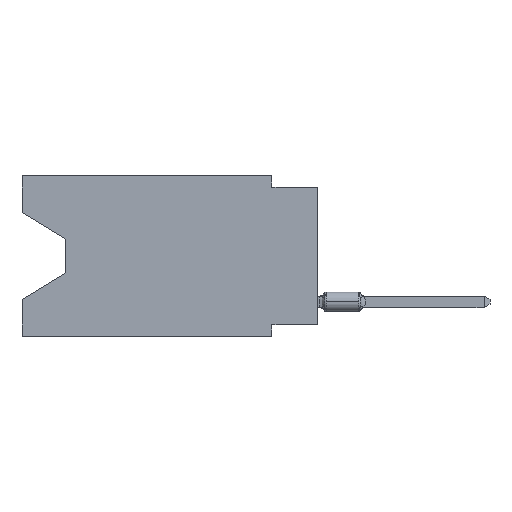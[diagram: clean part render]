
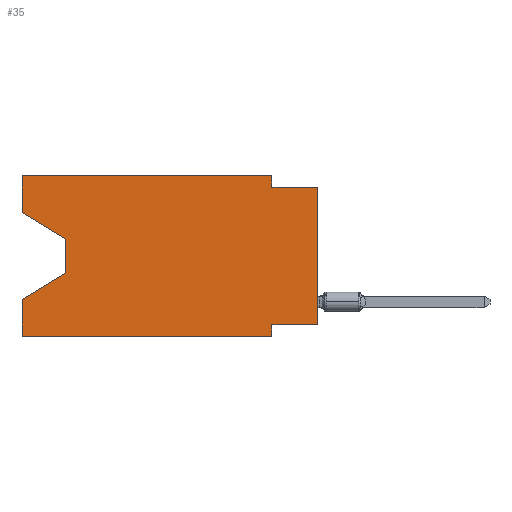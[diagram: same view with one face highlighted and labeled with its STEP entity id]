
A CAD part, left-side view. The second image highlights one B-rep face of the part: STEP entity #35.
In plain terms, the highlighted planar face has unit normal (-1, 0, 0).
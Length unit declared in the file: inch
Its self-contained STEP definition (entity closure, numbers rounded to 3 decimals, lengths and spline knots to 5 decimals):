
#35 = ADVANCED_FACE ( 'NONE', ( #199 ), #6060, .F. ) ;
#199 = FACE_OUTER_BOUND ( 'NONE', #285, .T. ) ;
#207 = VECTOR ( 'NONE', #5463, 39.37008 ) ;
#285 = EDGE_LOOP ( 'NONE', ( #1194, #2487, #8710, #9950, #14336, #1854, #3718, #14926, #2462, #6976, #872, #2185 ) ) ;
#323 = VECTOR ( 'NONE', #14289, 39.37008 ) ;
#442 = LINE ( 'NONE', #12983, #7200 ) ;
#547 = CARTESIAN_POINT ( 'NONE',  ( 0., 0.1, 0. ) ) ;
#564 = CARTESIAN_POINT ( 'NONE',  ( 0., 0.645, 0. ) ) ;
#569 = VERTEX_POINT ( 'NONE', #8991 ) ;
#685 = VECTOR ( 'NONE', #10960, 39.37008 ) ;
#872 = ORIENTED_EDGE ( 'NONE', *, *, #5659, .F. ) ;
#1194 = ORIENTED_EDGE ( 'NONE', *, *, #13750, .T. ) ;
#1289 = CARTESIAN_POINT ( 'NONE',  ( 0., 0., -0.325 ) ) ;
#1396 = LINE ( 'NONE', #14093, #13745 ) ;
#1601 = LINE ( 'NONE', #2672, #9532 ) ;
#1622 = DIRECTION ( 'NONE',  ( 0., 0., 1. ) ) ;
#1655 = DIRECTION ( 'NONE',  ( 0., 0., 1. ) ) ;
#1800 = VECTOR ( 'NONE', #10485, 39.37008 ) ;
#1826 = LINE ( 'NONE', #8537, #685 ) ;
#1854 = ORIENTED_EDGE ( 'NONE', *, *, #6015, .F. ) ;
#1916 = EDGE_CURVE ( 'NONE', #7897, #9151, #1601, .T. ) ;
#2185 = ORIENTED_EDGE ( 'NONE', *, *, #3210, .F. ) ;
#2310 = CARTESIAN_POINT ( 'NONE',  ( 0., 0.645, -0.35 ) ) ;
#2462 = ORIENTED_EDGE ( 'NONE', *, *, #7798, .F. ) ;
#2487 = ORIENTED_EDGE ( 'NONE', *, *, #11870, .T. ) ;
#2672 = CARTESIAN_POINT ( 'NONE',  ( 0., 0., -0.325 ) ) ;
#2851 = LINE ( 'NONE', #564, #5051 ) ;
#3210 = EDGE_CURVE ( 'NONE', #569, #8963, #8355, .T. ) ;
#3262 = DIRECTION ( 'NONE',  ( 0., -0.855, -0.519 ) ) ;
#3718 = ORIENTED_EDGE ( 'NONE', *, *, #1916, .F. ) ;
#3863 = DIRECTION ( 'NONE',  ( 1., 0., 0. ) ) ;
#3877 = CARTESIAN_POINT ( 'NONE',  ( 0., 0.1, -0.35 ) ) ;
#3897 = VERTEX_POINT ( 'NONE', #11573 ) ;
#4515 = EDGE_CURVE ( 'NONE', #5118, #12363, #7208, .T. ) ;
#5051 = VECTOR ( 'NONE', #1622, 39.37008 ) ;
#5079 = CARTESIAN_POINT ( 'NONE',  ( 0., 0.645, 0. ) ) ;
#5118 = VERTEX_POINT ( 'NONE', #2310 ) ;
#5463 = DIRECTION ( 'NONE',  ( 0., 0., -1. ) ) ;
#5659 = EDGE_CURVE ( 'NONE', #8963, #6902, #9208, .T. ) ;
#5695 = VERTEX_POINT ( 'NONE', #6234 ) ;
#6015 = EDGE_CURVE ( 'NONE', #9151, #12363, #12676, .T. ) ;
#6060 = PLANE ( 'NONE',  #7201 ) ;
#6234 = CARTESIAN_POINT ( 'NONE',  ( 0., 0.55, -0.212 ) ) ;
#6272 = VERTEX_POINT ( 'NONE', #9863 ) ;
#6749 = LINE ( 'NONE', #8810, #207 ) ;
#6893 = CARTESIAN_POINT ( 'NONE',  ( 0., 0.1, -0.35 ) ) ;
#6902 = VERTEX_POINT ( 'NONE', #547 ) ;
#6976 = ORIENTED_EDGE ( 'NONE', *, *, #12416, .F. ) ;
#7200 = VECTOR ( 'NONE', #1655, 39.37008 ) ;
#7201 = AXIS2_PLACEMENT_3D ( 'NONE', #5079, #3863, #14353 ) ;
#7208 = LINE ( 'NONE', #11852, #13923 ) ;
#7536 = EDGE_CURVE ( 'NONE', #5695, #6272, #1396, .T. ) ;
#7741 = VERTEX_POINT ( 'NONE', #12568 ) ;
#7798 = EDGE_CURVE ( 'NONE', #3897, #7741, #8850, .T. ) ;
#7897 = VERTEX_POINT ( 'NONE', #1289 ) ;
#8237 = CARTESIAN_POINT ( 'NONE',  ( 0., 0.1, -0.325 ) ) ;
#8319 = DIRECTION ( 'NONE',  ( 0., 0.855, -0.519 ) ) ;
#8355 = LINE ( 'NONE', #8438, #323 ) ;
#8438 = CARTESIAN_POINT ( 'NONE',  ( 0., 0.645, 0. ) ) ;
#8537 = CARTESIAN_POINT ( 'NONE',  ( 0., 0.55, -0.138 ) ) ;
#8710 = ORIENTED_EDGE ( 'NONE', *, *, #7536, .T. ) ;
#8810 = CARTESIAN_POINT ( 'NONE',  ( 0., 0.1, 0. ) ) ;
#8850 = LINE ( 'NONE', #13695, #11807 ) ;
#8963 = VERTEX_POINT ( 'NONE', #13559 ) ;
#8991 = CARTESIAN_POINT ( 'NONE',  ( 0., 0.645, -0.08025 ) ) ;
#9151 = VERTEX_POINT ( 'NONE', #8237 ) ;
#9208 = LINE ( 'NONE', #11778, #1800 ) ;
#9532 = VECTOR ( 'NONE', #9817, 39.37008 ) ;
#9817 = DIRECTION ( 'NONE',  ( 0., 1., 0. ) ) ;
#9863 = CARTESIAN_POINT ( 'NONE',  ( 0., 0.645, -0.26975 ) ) ;
#9950 = ORIENTED_EDGE ( 'NONE', *, *, #11453, .F. ) ;
#10073 = EDGE_CURVE ( 'NONE', #7897, #7741, #442, .T. ) ;
#10327 = CARTESIAN_POINT ( 'NONE',  ( 0., 0.645, -0.08025 ) ) ;
#10485 = DIRECTION ( 'NONE',  ( 0., -1., 0. ) ) ;
#10518 = CARTESIAN_POINT ( 'NONE',  ( 0., 0.55, -0.138 ) ) ;
#10706 = DIRECTION ( 'NONE',  ( 0., -1., 0. ) ) ;
#10960 = DIRECTION ( 'NONE',  ( 0., 0., -1. ) ) ;
#11453 = EDGE_CURVE ( 'NONE', #5118, #6272, #2851, .T. ) ;
#11539 = DIRECTION ( 'NONE',  ( 0., 0., -1. ) ) ;
#11573 = CARTESIAN_POINT ( 'NONE',  ( 0., 0.1, -0.025 ) ) ;
#11778 = CARTESIAN_POINT ( 'NONE',  ( 0., 0.645, 0. ) ) ;
#11807 = VECTOR ( 'NONE', #12413, 39.37008 ) ;
#11852 = CARTESIAN_POINT ( 'NONE',  ( 0., 0.645, -0.35 ) ) ;
#11870 = EDGE_CURVE ( 'NONE', #14970, #5695, #1826, .T. ) ;
#12363 = VERTEX_POINT ( 'NONE', #3877 ) ;
#12413 = DIRECTION ( 'NONE',  ( 0., -1., 0. ) ) ;
#12416 = EDGE_CURVE ( 'NONE', #6902, #3897, #6749, .T. ) ;
#12501 = VECTOR ( 'NONE', #11539, 39.37008 ) ;
#12568 = CARTESIAN_POINT ( 'NONE',  ( 0., 0., -0.025 ) ) ;
#12676 = LINE ( 'NONE', #6893, #12501 ) ;
#12679 = LINE ( 'NONE', #10327, #14080 ) ;
#12983 = CARTESIAN_POINT ( 'NONE',  ( 0., 0., 0. ) ) ;
#13559 = CARTESIAN_POINT ( 'NONE',  ( 0., 0.645, 0. ) ) ;
#13695 = CARTESIAN_POINT ( 'NONE',  ( 0., 0., -0.025 ) ) ;
#13745 = VECTOR ( 'NONE', #8319, 39.37008 ) ;
#13750 = EDGE_CURVE ( 'NONE', #569, #14970, #12679, .T. ) ;
#13923 = VECTOR ( 'NONE', #10706, 39.37008 ) ;
#14080 = VECTOR ( 'NONE', #3262, 39.37008 ) ;
#14093 = CARTESIAN_POINT ( 'NONE',  ( 0., 0.55, -0.212 ) ) ;
#14289 = DIRECTION ( 'NONE',  ( 0., 0., 1. ) ) ;
#14336 = ORIENTED_EDGE ( 'NONE', *, *, #4515, .T. ) ;
#14353 = DIRECTION ( 'NONE',  ( 0., 0., -1. ) ) ;
#14926 = ORIENTED_EDGE ( 'NONE', *, *, #10073, .T. ) ;
#14970 = VERTEX_POINT ( 'NONE', #10518 ) ;
